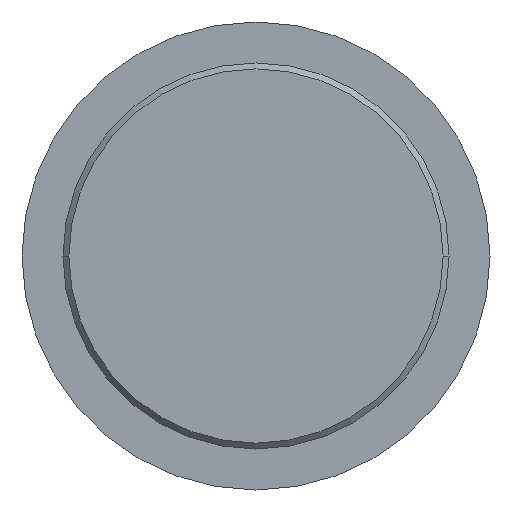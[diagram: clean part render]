
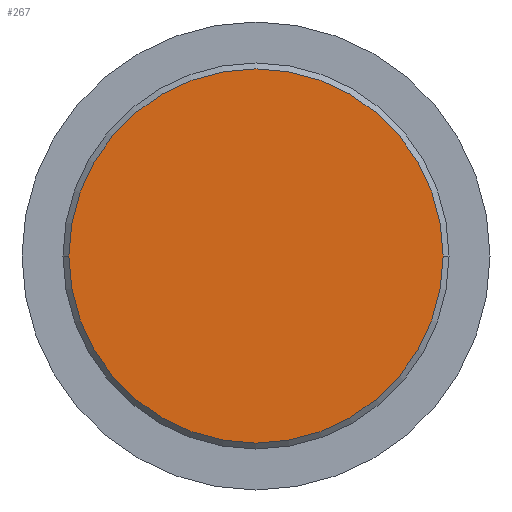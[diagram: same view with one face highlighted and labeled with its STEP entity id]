
A CAD part, front view. The second image highlights one B-rep face of the part: STEP entity #267.
In plain terms, the highlighted planar face has unit normal (0, -1, 0).
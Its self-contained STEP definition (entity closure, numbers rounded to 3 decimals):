
#6 = FACE_OUTER_BOUND ( 'NONE', #18, .T. ) ;
#18 = EDGE_LOOP ( 'NONE', ( #31, #37 ) ) ;
#31 = ORIENTED_EDGE ( 'NONE', *, *, #239, .F. ) ;
#37 = ORIENTED_EDGE ( 'NONE', *, *, #199, .F. ) ;
#43 = CIRCLE ( 'NONE', #176, 2.407 ) ;
#63 = CIRCLE ( 'NONE', #207, 2.407 ) ;
#98 = DIRECTION ( 'NONE',  ( 0., 0., -1. ) ) ;
#100 = DIRECTION ( 'NONE',  ( 0., -1., 0. ) ) ;
#102 = PLANE ( 'NONE',  #107 ) ;
#103 = CARTESIAN_POINT ( 'NONE',  ( -2.407, -11.656, 0. ) ) ;
#107 = AXIS2_PLACEMENT_3D ( 'NONE', #121, #100, #98 ) ;
#118 = DIRECTION ( 'NONE',  ( 1., 0., 0. ) ) ;
#119 = DIRECTION ( 'NONE',  ( 0., 1., 0. ) ) ;
#120 = CARTESIAN_POINT ( 'NONE',  ( 0., -11.656, 0. ) ) ;
#121 = CARTESIAN_POINT ( 'NONE',  ( 0., -11.656, 0. ) ) ;
#123 = VERTEX_POINT ( 'NONE', #263 ) ;
#157 = DIRECTION ( 'NONE',  ( 1., 0., 0. ) ) ;
#158 = DIRECTION ( 'NONE',  ( 0., 1., 0. ) ) ;
#160 = CARTESIAN_POINT ( 'NONE',  ( 0., -11.656, 0. ) ) ;
#176 = AXIS2_PLACEMENT_3D ( 'NONE', #120, #119, #118 ) ;
#199 = EDGE_CURVE ( 'NONE', #266, #123, #63, .T. ) ;
#207 = AXIS2_PLACEMENT_3D ( 'NONE', #160, #158, #157 ) ;
#239 = EDGE_CURVE ( 'NONE', #123, #266, #43, .T. ) ;
#263 = CARTESIAN_POINT ( 'NONE',  ( 2.407, -11.656, 0. ) ) ;
#266 = VERTEX_POINT ( 'NONE', #103 ) ;
#267 = ADVANCED_FACE ( 'NONE', ( #6 ), #102, .T. ) ;
